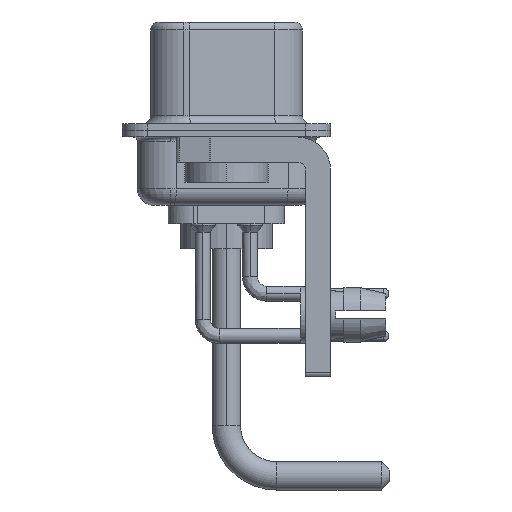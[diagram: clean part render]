
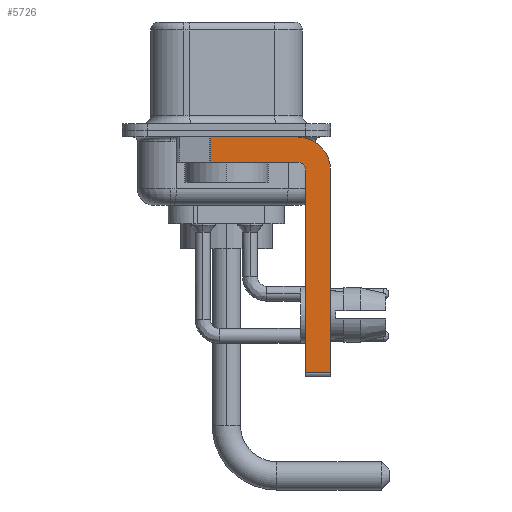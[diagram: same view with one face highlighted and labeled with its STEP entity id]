
A CAD part, left-side view. The second image highlights one B-rep face of the part: STEP entity #5726.
In plain terms, the highlighted planar face has unit normal (-1, 0, 0).
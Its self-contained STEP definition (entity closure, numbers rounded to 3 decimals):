
#110 = ORIENTED_EDGE ( 'NONE', *, *, #708, .F. ) ;
#240 = DIRECTION ( 'NONE',  ( 1., 0., 0. ) ) ;
#519 = CARTESIAN_POINT ( 'NONE',  ( -2.9, -4.25, -2.4 ) ) ;
#708 = EDGE_CURVE ( 'NONE', #15194, #25946, #6693, .T. ) ;
#822 = CARTESIAN_POINT ( 'NONE',  ( -2.9, -4.75, -14.55 ) ) ;
#1229 = VERTEX_POINT ( 'NONE', #822 ) ;
#1259 = VECTOR ( 'NONE', #21883, 1000. ) ;
#1346 = ORIENTED_EDGE ( 'NONE', *, *, #17306, .F. ) ;
#2521 = CARTESIAN_POINT ( 'NONE',  ( -2.9, -4.25, -14.55 ) ) ;
#2583 = LINE ( 'NONE', #18142, #22958 ) ;
#3060 = VECTOR ( 'NONE', #28264, 1000. ) ;
#5004 = VERTEX_POINT ( 'NONE', #15428 ) ;
#5129 = LINE ( 'NONE', #2521, #5509 ) ;
#5222 = ORIENTED_EDGE ( 'NONE', *, *, #21126, .T. ) ;
#5509 = VECTOR ( 'NONE', #7296, 1000. ) ;
#5690 = CARTESIAN_POINT ( 'NONE',  ( -2.9, 0.978, -1.9 ) ) ;
#5726 = ADVANCED_FACE ( 'NONE', ( #16906 ), #23170, .F. ) ;
#5955 = LINE ( 'NONE', #14735, #14856 ) ;
#6432 = VECTOR ( 'NONE', #12327, 1000. ) ;
#6693 = LINE ( 'NONE', #23617, #1259 ) ;
#7186 = DIRECTION ( 'NONE',  ( 0., 0., -1. ) ) ;
#7296 = DIRECTION ( 'NONE',  ( 0., -1., 0. ) ) ;
#7846 = DIRECTION ( 'NONE',  ( 0., 0., -1. ) ) ;
#7982 = DIRECTION ( 'NONE',  ( 1., 0., 0. ) ) ;
#7993 = CARTESIAN_POINT ( 'NONE',  ( -2.9, -4.25, -0.4 ) ) ;
#8126 = CARTESIAN_POINT ( 'NONE',  ( -2.9, -4.25, -2.4 ) ) ;
#8579 = EDGE_CURVE ( 'NONE', #1229, #5004, #5129, .T. ) ;
#10481 = LINE ( 'NONE', #27841, #3060 ) ;
#10669 = EDGE_CURVE ( 'NONE', #15485, #24498, #2583, .T. ) ;
#10747 = ORIENTED_EDGE ( 'NONE', *, *, #17867, .F. ) ;
#10983 = CARTESIAN_POINT ( 'NONE',  ( -2.9, -4.25, -2.4 ) ) ;
#11378 = AXIS2_PLACEMENT_3D ( 'NONE', #519, #240, #7186 ) ;
#11714 = CARTESIAN_POINT ( 'NONE',  ( -2.9, -6.25, -2.4 ) ) ;
#12327 = DIRECTION ( 'NONE',  ( 0., 0., -1. ) ) ;
#12827 = CARTESIAN_POINT ( 'NONE',  ( -2.9, -4.25, -1.9 ) ) ;
#12982 = DIRECTION ( 'NONE',  ( 0., 0., 1. ) ) ;
#13026 = AXIS2_PLACEMENT_3D ( 'NONE', #8126, #7982, #7846 ) ;
#14274 = EDGE_LOOP ( 'NONE', ( #110, #5222, #17682, #1346, #14278, #25196, #26748, #10747 ) ) ;
#14278 = ORIENTED_EDGE ( 'NONE', *, *, #22655, .F. ) ;
#14494 = VERTEX_POINT ( 'NONE', #27803 ) ;
#14735 = CARTESIAN_POINT ( 'NONE',  ( -2.9, -4.75, -14.8 ) ) ;
#14856 = VECTOR ( 'NONE', #23436, 1000. ) ;
#15194 = VERTEX_POINT ( 'NONE', #26179 ) ;
#15428 = CARTESIAN_POINT ( 'NONE',  ( -2.9, -6.25, -14.55 ) ) ;
#15485 = VERTEX_POINT ( 'NONE', #12827 ) ;
#15709 = DIRECTION ( 'NONE',  ( 0., 1., 0. ) ) ;
#16906 = FACE_OUTER_BOUND ( 'NONE', #14274, .T. ) ;
#17306 = EDGE_CURVE ( 'NONE', #14494, #15485, #22295, .T. ) ;
#17682 = ORIENTED_EDGE ( 'NONE', *, *, #10669, .F. ) ;
#17867 = EDGE_CURVE ( 'NONE', #25946, #22720, #28289, .T. ) ;
#18142 = CARTESIAN_POINT ( 'NONE',  ( -2.9, -4.25, -1.9 ) ) ;
#18186 = EDGE_CURVE ( 'NONE', #22720, #5004, #10481, .T. ) ;
#19565 = DIRECTION ( 'NONE',  ( -1., 0., 0. ) ) ;
#21126 = EDGE_CURVE ( 'NONE', #15194, #24498, #25356, .T. ) ;
#21883 = DIRECTION ( 'NONE',  ( 0., -1., 0. ) ) ;
#22295 = CIRCLE ( 'NONE', #23186, 0.5 ) ;
#22655 = EDGE_CURVE ( 'NONE', #1229, #14494, #5955, .T. ) ;
#22720 = VERTEX_POINT ( 'NONE', #11714 ) ;
#22958 = VECTOR ( 'NONE', #15709, 1000. ) ;
#23097 = CARTESIAN_POINT ( 'NONE',  ( -2.9, 0.978, -1.9 ) ) ;
#23170 = PLANE ( 'NONE',  #13026 ) ;
#23186 = AXIS2_PLACEMENT_3D ( 'NONE', #10983, #19565, #12982 ) ;
#23436 = DIRECTION ( 'NONE',  ( 0., 0., 1. ) ) ;
#23617 = CARTESIAN_POINT ( 'NONE',  ( -2.9, 3., -0.4 ) ) ;
#24498 = VERTEX_POINT ( 'NONE', #23097 ) ;
#25196 = ORIENTED_EDGE ( 'NONE', *, *, #8579, .T. ) ;
#25356 = LINE ( 'NONE', #5690, #6432 ) ;
#25946 = VERTEX_POINT ( 'NONE', #7993 ) ;
#26179 = CARTESIAN_POINT ( 'NONE',  ( -2.9, 0.978, -0.4 ) ) ;
#26748 = ORIENTED_EDGE ( 'NONE', *, *, #18186, .F. ) ;
#27803 = CARTESIAN_POINT ( 'NONE',  ( -2.9, -4.75, -2.4 ) ) ;
#27841 = CARTESIAN_POINT ( 'NONE',  ( -2.9, -6.25, -2.4 ) ) ;
#28264 = DIRECTION ( 'NONE',  ( 0., 0., -1. ) ) ;
#28289 = CIRCLE ( 'NONE', #11378, 2. ) ;
